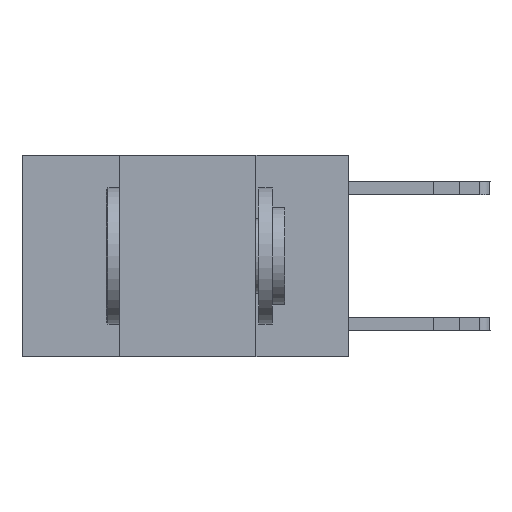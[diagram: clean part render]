
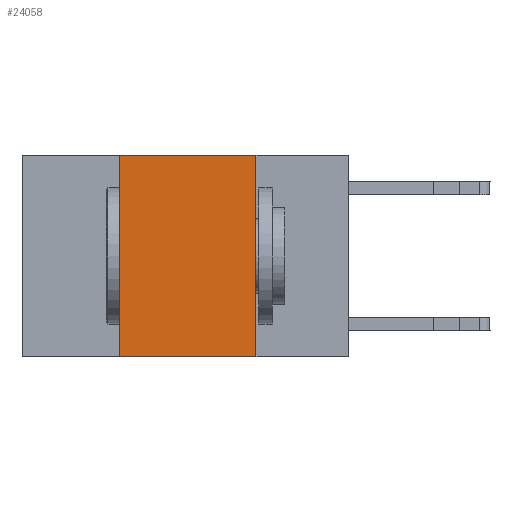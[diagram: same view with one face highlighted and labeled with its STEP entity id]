
A CAD part, left-side view. The second image highlights one B-rep face of the part: STEP entity #24058.
In plain terms, the highlighted planar face has unit normal (-1, 0, 0).
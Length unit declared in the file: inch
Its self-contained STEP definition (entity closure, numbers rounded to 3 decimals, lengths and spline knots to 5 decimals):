
#301 = VERTEX_POINT ( 'NONE', #1659 ) ;
#411 = DIRECTION ( 'NONE',  ( 0., 0., -1. ) ) ;
#1659 = CARTESIAN_POINT ( 'NONE',  ( 0., 0.17, 0. ) ) ;
#1923 = DIRECTION ( 'NONE',  ( 0., 0., 1. ) ) ;
#3275 = VECTOR ( 'NONE', #21640, 39.37008 ) ;
#5453 = LINE ( 'NONE', #17242, #23217 ) ;
#6760 = EDGE_CURVE ( 'NONE', #7465, #301, #5453, .T. ) ;
#7147 = ORIENTED_EDGE ( 'NONE', *, *, #12075, .T. ) ;
#7465 = VERTEX_POINT ( 'NONE', #12603 ) ;
#9339 = EDGE_LOOP ( 'NONE', ( #24407, #23092, #16987, #7147 ) ) ;
#9401 = LINE ( 'NONE', #19250, #10635 ) ;
#9521 = VERTEX_POINT ( 'NONE', #12852 ) ;
#10635 = VECTOR ( 'NONE', #1923, 39.37008 ) ;
#11534 = VECTOR ( 'NONE', #16372, 39.37008 ) ;
#11890 = CARTESIAN_POINT ( 'NONE',  ( 0., 0.6, 0. ) ) ;
#12075 = EDGE_CURVE ( 'NONE', #14048, #9521, #23755, .T. ) ;
#12603 = CARTESIAN_POINT ( 'NONE',  ( 0., 0.42, 0. ) ) ;
#12852 = CARTESIAN_POINT ( 'NONE',  ( 0., 0.17, -0.37 ) ) ;
#13219 = EDGE_CURVE ( 'NONE', #14048, #7465, #9401, .T. ) ;
#13787 = FACE_OUTER_BOUND ( 'NONE', #9339, .T. ) ;
#14048 = VERTEX_POINT ( 'NONE', #16575 ) ;
#14203 = AXIS2_PLACEMENT_3D ( 'NONE', #11890, #17723, #411 ) ;
#15349 = DIRECTION ( 'NONE',  ( 0., -1., 0. ) ) ;
#16372 = DIRECTION ( 'NONE',  ( 0., 0., -1. ) ) ;
#16575 = CARTESIAN_POINT ( 'NONE',  ( 0., 0.42, -0.37 ) ) ;
#16987 = ORIENTED_EDGE ( 'NONE', *, *, #13219, .F. ) ;
#17242 = CARTESIAN_POINT ( 'NONE',  ( 0., 0.6, 0. ) ) ;
#17723 = DIRECTION ( 'NONE',  ( 1., 0., 0. ) ) ;
#18300 = EDGE_CURVE ( 'NONE', #301, #9521, #21924, .T. ) ;
#19250 = CARTESIAN_POINT ( 'NONE',  ( 0., 0.42, 0. ) ) ;
#21490 = PLANE ( 'NONE',  #14203 ) ;
#21640 = DIRECTION ( 'NONE',  ( 0., -1., 0. ) ) ;
#21881 = CARTESIAN_POINT ( 'NONE',  ( 0., 0.6, -0.37 ) ) ;
#21924 = LINE ( 'NONE', #22169, #11534 ) ;
#22169 = CARTESIAN_POINT ( 'NONE',  ( 0., 0.17, 0. ) ) ;
#23092 = ORIENTED_EDGE ( 'NONE', *, *, #6760, .F. ) ;
#23217 = VECTOR ( 'NONE', #15349, 39.37008 ) ;
#23755 = LINE ( 'NONE', #21881, #3275 ) ;
#24058 = ADVANCED_FACE ( 'NONE', ( #13787 ), #21490, .F. ) ;
#24407 = ORIENTED_EDGE ( 'NONE', *, *, #18300, .F. ) ;
